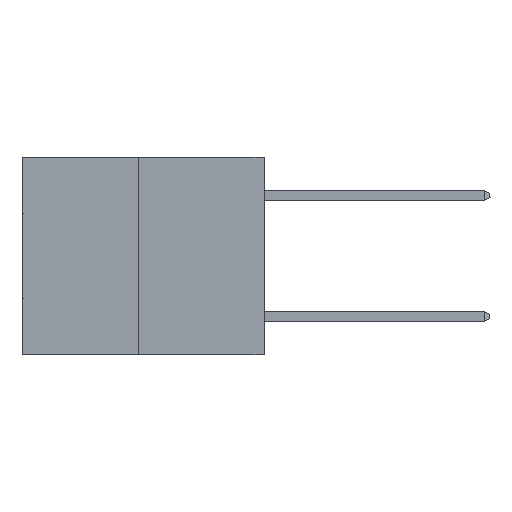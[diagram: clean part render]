
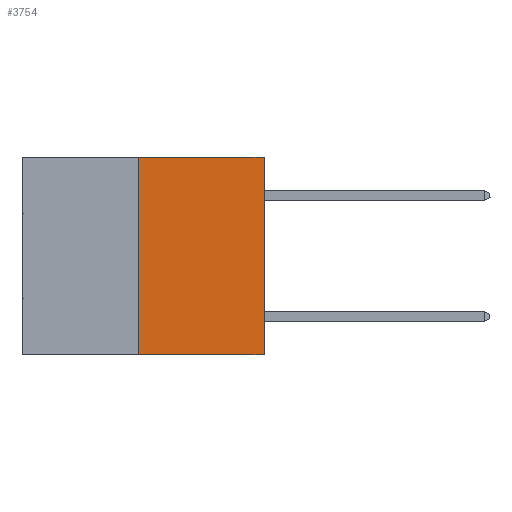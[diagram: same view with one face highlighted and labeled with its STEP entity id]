
A CAD part, left-side view. The second image highlights one B-rep face of the part: STEP entity #3754.
In plain terms, the highlighted planar face has unit normal (-1, 0, 0).
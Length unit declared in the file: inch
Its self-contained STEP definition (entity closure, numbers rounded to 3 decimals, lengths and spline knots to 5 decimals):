
#390 = CARTESIAN_POINT ( 'NONE',  ( 0., 0., -0.49 ) ) ;
#1946 = DIRECTION ( 'NONE',  ( 0., 0., 1. ) ) ;
#2385 = VERTEX_POINT ( 'NONE', #4818 ) ;
#2805 = EDGE_CURVE ( 'NONE', #18334, #2385, #8928, .T. ) ;
#3306 = LINE ( 'NONE', #7899, #19839 ) ;
#3691 = VECTOR ( 'NONE', #1946, 39.37008 ) ;
#3754 = ADVANCED_FACE ( 'NONE', ( #32285 ), #20157, .F. ) ;
#4686 = CARTESIAN_POINT ( 'NONE',  ( 0., 0.6, 0. ) ) ;
#4818 = CARTESIAN_POINT ( 'NONE',  ( 0., 0., 0. ) ) ;
#6893 = ORIENTED_EDGE ( 'NONE', *, *, #17468, .T. ) ;
#6924 = LINE ( 'NONE', #6997, #3691 ) ;
#6997 = CARTESIAN_POINT ( 'NONE',  ( 0., 0.312, -0.49 ) ) ;
#7376 = VECTOR ( 'NONE', #11897, 39.37008 ) ;
#7899 = CARTESIAN_POINT ( 'NONE',  ( 0., 0., 0. ) ) ;
#8310 = CARTESIAN_POINT ( 'NONE',  ( 0., 0.312, -0.49 ) ) ;
#8928 = LINE ( 'NONE', #26979, #21451 ) ;
#8974 = CARTESIAN_POINT ( 'NONE',  ( 0., 0.6, -0.49 ) ) ;
#11270 = CARTESIAN_POINT ( 'NONE',  ( 0., 0.312, 0. ) ) ;
#11897 = DIRECTION ( 'NONE',  ( 0., -1., 0. ) ) ;
#13620 = EDGE_LOOP ( 'NONE', ( #25609, #6893, #24248, #20472 ) ) ;
#16056 = VERTEX_POINT ( 'NONE', #8310 ) ;
#17468 = EDGE_CURVE ( 'NONE', #16056, #25276, #19915, .T. ) ;
#18334 = VERTEX_POINT ( 'NONE', #11270 ) ;
#19839 = VECTOR ( 'NONE', #33289, 39.37008 ) ;
#19915 = LINE ( 'NONE', #8974, #7376 ) ;
#20157 = PLANE ( 'NONE',  #23533 ) ;
#20472 = ORIENTED_EDGE ( 'NONE', *, *, #2805, .F. ) ;
#21451 = VECTOR ( 'NONE', #24517, 39.37008 ) ;
#22045 = EDGE_CURVE ( 'NONE', #16056, #18334, #6924, .T. ) ;
#22303 = DIRECTION ( 'NONE',  ( 0., 0., -1. ) ) ;
#23533 = AXIS2_PLACEMENT_3D ( 'NONE', #4686, #29957, #22303 ) ;
#24248 = ORIENTED_EDGE ( 'NONE', *, *, #30050, .T. ) ;
#24517 = DIRECTION ( 'NONE',  ( 0., -1., 0. ) ) ;
#25276 = VERTEX_POINT ( 'NONE', #390 ) ;
#25609 = ORIENTED_EDGE ( 'NONE', *, *, #22045, .F. ) ;
#26979 = CARTESIAN_POINT ( 'NONE',  ( 0., 0.6, 0. ) ) ;
#29957 = DIRECTION ( 'NONE',  ( 1., 0., 0. ) ) ;
#30050 = EDGE_CURVE ( 'NONE', #25276, #2385, #3306, .T. ) ;
#32285 = FACE_OUTER_BOUND ( 'NONE', #13620, .T. ) ;
#33289 = DIRECTION ( 'NONE',  ( 0., 0., 1. ) ) ;
